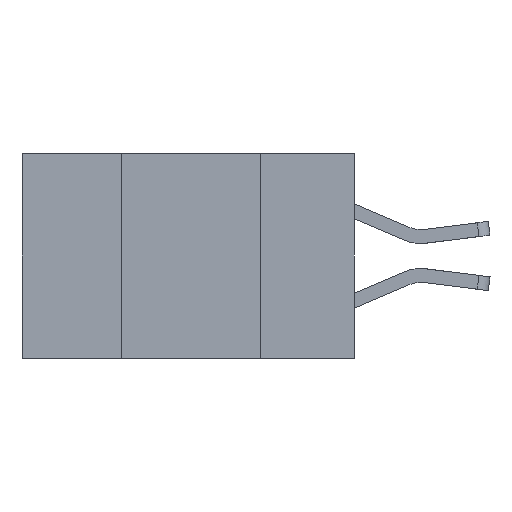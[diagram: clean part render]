
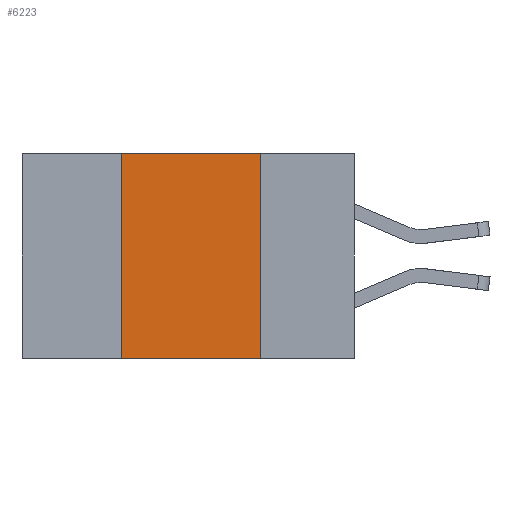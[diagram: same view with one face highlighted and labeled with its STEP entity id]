
A CAD part, left-side view. The second image highlights one B-rep face of the part: STEP entity #6223.
In plain terms, the highlighted planar face has unit normal (-1, 0, 0).
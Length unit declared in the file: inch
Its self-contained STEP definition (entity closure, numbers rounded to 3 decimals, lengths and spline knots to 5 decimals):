
#29 = ORIENTED_EDGE ( 'NONE', *, *, #9067, .F. ) ;
#319 = ORIENTED_EDGE ( 'NONE', *, *, #7139, .T. ) ;
#555 = CARTESIAN_POINT ( 'NONE',  ( 0., 0.6, 0. ) ) ;
#641 = DIRECTION ( 'NONE',  ( 0., -1., 0. ) ) ;
#696 = VERTEX_POINT ( 'NONE', #3218 ) ;
#730 = VECTOR ( 'NONE', #1739, 39.37008 ) ;
#1208 = DIRECTION ( 'NONE',  ( 0., 0., -1. ) ) ;
#1581 = CARTESIAN_POINT ( 'NONE',  ( 0., 0.42, 0. ) ) ;
#1739 = DIRECTION ( 'NONE',  ( 0., 0., -1. ) ) ;
#2031 = CARTESIAN_POINT ( 'NONE',  ( 0., 0.17, 0. ) ) ;
#2116 = ORIENTED_EDGE ( 'NONE', *, *, #9049, .F. ) ;
#2863 = DIRECTION ( 'NONE',  ( 0., -1., 0. ) ) ;
#3218 = CARTESIAN_POINT ( 'NONE',  ( 0., 0.17, -0.37 ) ) ;
#4007 = DIRECTION ( 'NONE',  ( 1., 0., 0. ) ) ;
#4108 = CARTESIAN_POINT ( 'NONE',  ( 0., 0.6, -0.37 ) ) ;
#4214 = LINE ( 'NONE', #9147, #8994 ) ;
#4238 = DIRECTION ( 'NONE',  ( 0., 0., 1. ) ) ;
#4287 = VERTEX_POINT ( 'NONE', #8670 ) ;
#4419 = EDGE_LOOP ( 'NONE', ( #29, #2116, #8249, #319 ) ) ;
#4480 = LINE ( 'NONE', #4108, #10236 ) ;
#4671 = VERTEX_POINT ( 'NONE', #9541 ) ;
#4756 = LINE ( 'NONE', #2031, #730 ) ;
#5915 = AXIS2_PLACEMENT_3D ( 'NONE', #555, #4007, #1208 ) ;
#6223 = ADVANCED_FACE ( 'NONE', ( #6413 ), #11287, .F. ) ;
#6413 = FACE_OUTER_BOUND ( 'NONE', #4419, .T. ) ;
#6921 = CARTESIAN_POINT ( 'NONE',  ( 0., 0.42, 0. ) ) ;
#7139 = EDGE_CURVE ( 'NONE', #4287, #696, #4480, .T. ) ;
#7745 = VERTEX_POINT ( 'NONE', #1581 ) ;
#8249 = ORIENTED_EDGE ( 'NONE', *, *, #11099, .F. ) ;
#8670 = CARTESIAN_POINT ( 'NONE',  ( 0., 0.42, -0.37 ) ) ;
#8994 = VECTOR ( 'NONE', #2863, 39.37008 ) ;
#9049 = EDGE_CURVE ( 'NONE', #7745, #4671, #4214, .T. ) ;
#9067 = EDGE_CURVE ( 'NONE', #4671, #696, #4756, .T. ) ;
#9147 = CARTESIAN_POINT ( 'NONE',  ( 0., 0.6, 0. ) ) ;
#9403 = LINE ( 'NONE', #6921, #9958 ) ;
#9541 = CARTESIAN_POINT ( 'NONE',  ( 0., 0.17, 0. ) ) ;
#9958 = VECTOR ( 'NONE', #4238, 39.37008 ) ;
#10236 = VECTOR ( 'NONE', #641, 39.37008 ) ;
#11099 = EDGE_CURVE ( 'NONE', #4287, #7745, #9403, .T. ) ;
#11287 = PLANE ( 'NONE',  #5915 ) ;
